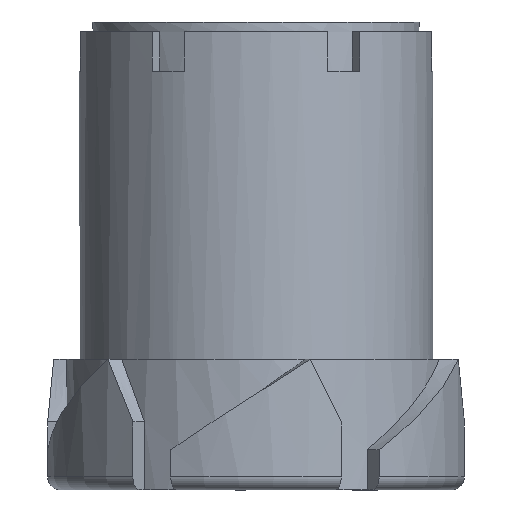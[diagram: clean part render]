
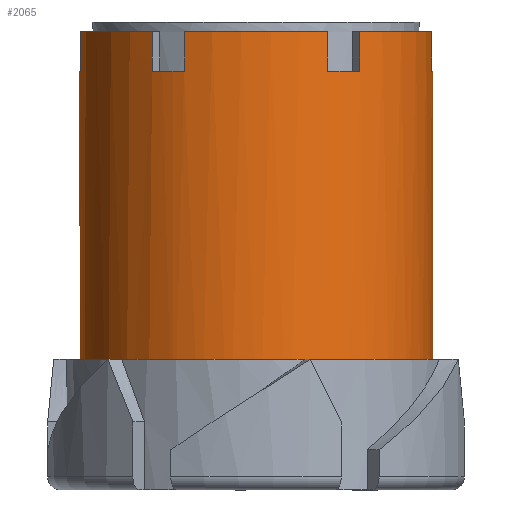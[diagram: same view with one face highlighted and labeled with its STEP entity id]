
A CAD part, left-side view. The second image highlights one B-rep face of the part: STEP entity #2065.
In plain terms, the highlighted cylindrical face has radius 27 mm (diameter 54 mm), a full revolution.
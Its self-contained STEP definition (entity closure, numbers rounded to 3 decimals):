
#1794=CARTESIAN_POINT('',(26.852,28.,-2.822));
#1795=VERTEX_POINT('',#1794);
#1802=CARTESIAN_POINT('',(26.852,34.0,-2.822));
#1803=VERTEX_POINT('',#1802);
#1804=CARTESIAN_POINT('',(26.852,34.0,-2.822));
#1805=DIRECTION('',(0.0,-1.0,0.0));
#1806=VECTOR('',#1805,6.);
#1807=LINE('',#1804,#1806);
#1808=EDGE_CURVE('',#1803,#1795,#1807,.T.);
#1833=CARTESIAN_POINT('',(15.87,34.0,-21.843));
#1834=VERTEX_POINT('',#1833);
#1835=CARTESIAN_POINT('',(0.0,34.0,0.0));
#1836=DIRECTION('',(0.0,-1.0,0.0));
#1837=DIRECTION('',(1.0,0.0,0.0));
#1838=AXIS2_PLACEMENT_3D('',#1835,#1836,#1837);
#1839=CIRCLE('',#1838,27.0);
#1840=EDGE_CURVE('',#1834,#1803,#1839,.T.);
#1860=CARTESIAN_POINT('',(0.0,0.0,0.0));
#1861=DIRECTION('',(0.0,1.0,0.0));
#1862=DIRECTION('',(1.0,0.0,0.0));
#1863=AXIS2_PLACEMENT_3D('',#1860,#1861,#1862);
#1864=CYLINDRICAL_SURFACE('',#1863,27.0);
#1865=CARTESIAN_POINT('',(-27.0,-36.0,0.));
#1866=VERTEX_POINT('',#1865);
#1867=CARTESIAN_POINT('',(0.0,-36.0,0.0));
#1868=DIRECTION('',(0.0,1.0,0.0));
#1869=DIRECTION('',(1.0,0.0,0.0));
#1870=AXIS2_PLACEMENT_3D('',#1867,#1868,#1869);
#1871=CIRCLE('',#1870,27.0);
#1872=EDGE_CURVE('',#1866,#1866,#1871,.T.);
#1873=ORIENTED_EDGE('',*,*,#1872,.T.);
#1874=EDGE_LOOP('',(#1873));
#1875=FACE_OUTER_BOUND('',#1874,.T.);
#1876=ORIENTED_EDGE('',*,*,#1808,.T.);
#1877=CARTESIAN_POINT('',(26.852,28.,2.822));
#1878=VERTEX_POINT('',#1877);
#1879=CARTESIAN_POINT('',(0.0,28.,0.0));
#1880=DIRECTION('',(0.0,-1.0,0.0));
#1881=DIRECTION('',(1.0,0.0,0.0));
#1882=AXIS2_PLACEMENT_3D('',#1879,#1880,#1881);
#1883=CIRCLE('',#1882,27.0);
#1884=EDGE_CURVE('',#1795,#1878,#1883,.T.);
#1885=ORIENTED_EDGE('',*,*,#1884,.T.);
#1886=CARTESIAN_POINT('',(26.852,34.0,2.822));
#1887=VERTEX_POINT('',#1886);
#1888=CARTESIAN_POINT('',(26.852,28.,2.822));
#1889=DIRECTION('',(0.0,1.0,0.0));
#1890=VECTOR('',#1889,6.);
#1891=LINE('',#1888,#1890);
#1892=EDGE_CURVE('',#1878,#1887,#1891,.T.);
#1893=ORIENTED_EDGE('',*,*,#1892,.T.);
#1894=CARTESIAN_POINT('',(15.87,34.0,21.843));
#1895=VERTEX_POINT('',#1894);
#1896=CARTESIAN_POINT('',(0.0,34.0,0.0));
#1897=DIRECTION('',(0.0,-1.0,0.0));
#1898=DIRECTION('',(1.0,0.0,0.0));
#1899=AXIS2_PLACEMENT_3D('',#1896,#1897,#1898);
#1900=CIRCLE('',#1899,27.0);
#1901=EDGE_CURVE('',#1887,#1895,#1900,.T.);
#1902=ORIENTED_EDGE('',*,*,#1901,.T.);
#1903=CARTESIAN_POINT('',(15.87,28.,21.843));
#1904=VERTEX_POINT('',#1903);
#1905=CARTESIAN_POINT('',(15.87,34.0,21.843));
#1906=DIRECTION('',(0.0,-1.0,0.0));
#1907=VECTOR('',#1906,6.);
#1908=LINE('',#1905,#1907);
#1909=EDGE_CURVE('',#1895,#1904,#1908,.T.);
#1910=ORIENTED_EDGE('',*,*,#1909,.T.);
#1911=CARTESIAN_POINT('',(10.982,28.,24.666));
#1912=VERTEX_POINT('',#1911);
#1913=CARTESIAN_POINT('',(0.0,28.,0.0));
#1914=DIRECTION('',(0.0,-1.0,0.0));
#1915=DIRECTION('',(1.0,0.0,0.0));
#1916=AXIS2_PLACEMENT_3D('',#1913,#1914,#1915);
#1917=CIRCLE('',#1916,27.0);
#1918=EDGE_CURVE('',#1904,#1912,#1917,.T.);
#1919=ORIENTED_EDGE('',*,*,#1918,.T.);
#1920=CARTESIAN_POINT('',(10.982,34.0,24.666));
#1921=VERTEX_POINT('',#1920);
#1922=CARTESIAN_POINT('',(10.982,28.,24.666));
#1923=DIRECTION('',(0.0,1.0,0.0));
#1924=VECTOR('',#1923,6.);
#1925=LINE('',#1922,#1924);
#1926=EDGE_CURVE('',#1912,#1921,#1925,.T.);
#1927=ORIENTED_EDGE('',*,*,#1926,.T.);
#1928=CARTESIAN_POINT('',(-10.982,34.0,24.666));
#1929=VERTEX_POINT('',#1928);
#1930=CARTESIAN_POINT('',(0.0,34.0,0.0));
#1931=DIRECTION('',(0.0,-1.0,0.0));
#1932=DIRECTION('',(1.0,0.0,0.0));
#1933=AXIS2_PLACEMENT_3D('',#1930,#1931,#1932);
#1934=CIRCLE('',#1933,27.0);
#1935=EDGE_CURVE('',#1921,#1929,#1934,.T.);
#1936=ORIENTED_EDGE('',*,*,#1935,.T.);
#1937=CARTESIAN_POINT('',(-10.982,28.,24.666));
#1938=VERTEX_POINT('',#1937);
#1939=CARTESIAN_POINT('',(-10.982,34.0,24.666));
#1940=DIRECTION('',(0.0,-1.0,0.0));
#1941=VECTOR('',#1940,6.);
#1942=LINE('',#1939,#1941);
#1943=EDGE_CURVE('',#1929,#1938,#1942,.T.);
#1944=ORIENTED_EDGE('',*,*,#1943,.T.);
#1945=CARTESIAN_POINT('',(-15.87,28.,21.843));
#1946=VERTEX_POINT('',#1945);
#1947=CARTESIAN_POINT('',(0.0,28.,0.0));
#1948=DIRECTION('',(0.0,-1.0,0.0));
#1949=DIRECTION('',(1.0,0.0,0.0));
#1950=AXIS2_PLACEMENT_3D('',#1947,#1948,#1949);
#1951=CIRCLE('',#1950,27.0);
#1952=EDGE_CURVE('',#1938,#1946,#1951,.T.);
#1953=ORIENTED_EDGE('',*,*,#1952,.T.);
#1954=CARTESIAN_POINT('',(-15.87,34.0,21.843));
#1955=VERTEX_POINT('',#1954);
#1956=CARTESIAN_POINT('',(-15.87,28.,21.843));
#1957=DIRECTION('',(0.0,1.0,0.0));
#1958=VECTOR('',#1957,6.);
#1959=LINE('',#1956,#1958);
#1960=EDGE_CURVE('',#1946,#1955,#1959,.T.);
#1961=ORIENTED_EDGE('',*,*,#1960,.T.);
#1962=CARTESIAN_POINT('',(-26.852,34.0,2.822));
#1963=VERTEX_POINT('',#1962);
#1964=CARTESIAN_POINT('',(0.0,34.0,0.0));
#1965=DIRECTION('',(0.0,-1.0,0.0));
#1966=DIRECTION('',(1.0,0.0,0.0));
#1967=AXIS2_PLACEMENT_3D('',#1964,#1965,#1966);
#1968=CIRCLE('',#1967,27.0);
#1969=EDGE_CURVE('',#1955,#1963,#1968,.T.);
#1970=ORIENTED_EDGE('',*,*,#1969,.T.);
#1971=CARTESIAN_POINT('',(-26.852,28.,2.822));
#1972=VERTEX_POINT('',#1971);
#1973=CARTESIAN_POINT('',(-26.852,34.0,2.822));
#1974=DIRECTION('',(0.0,-1.0,0.0));
#1975=VECTOR('',#1974,6.);
#1976=LINE('',#1973,#1975);
#1977=EDGE_CURVE('',#1963,#1972,#1976,.T.);
#1978=ORIENTED_EDGE('',*,*,#1977,.T.);
#1979=CARTESIAN_POINT('',(-26.852,28.,-2.822));
#1980=VERTEX_POINT('',#1979);
#1981=CARTESIAN_POINT('',(0.0,28.,0.0));
#1982=DIRECTION('',(0.0,-1.0,0.0));
#1983=DIRECTION('',(1.0,0.0,0.0));
#1984=AXIS2_PLACEMENT_3D('',#1981,#1982,#1983);
#1985=CIRCLE('',#1984,27.0);
#1986=EDGE_CURVE('',#1972,#1980,#1985,.T.);
#1987=ORIENTED_EDGE('',*,*,#1986,.T.);
#1988=CARTESIAN_POINT('',(-26.852,34.0,-2.822));
#1989=VERTEX_POINT('',#1988);
#1990=CARTESIAN_POINT('',(-26.852,28.,-2.822));
#1991=DIRECTION('',(0.0,1.0,0.0));
#1992=VECTOR('',#1991,6.);
#1993=LINE('',#1990,#1992);
#1994=EDGE_CURVE('',#1980,#1989,#1993,.T.);
#1995=ORIENTED_EDGE('',*,*,#1994,.T.);
#1996=CARTESIAN_POINT('',(-15.87,34.0,-21.843));
#1997=VERTEX_POINT('',#1996);
#1998=CARTESIAN_POINT('',(0.0,34.0,0.0));
#1999=DIRECTION('',(0.0,-1.0,0.0));
#2000=DIRECTION('',(1.0,0.0,0.0));
#2001=AXIS2_PLACEMENT_3D('',#1998,#1999,#2000);
#2002=CIRCLE('',#2001,27.0);
#2003=EDGE_CURVE('',#1989,#1997,#2002,.T.);
#2004=ORIENTED_EDGE('',*,*,#2003,.T.);
#2005=CARTESIAN_POINT('',(-15.87,28.,-21.843));
#2006=VERTEX_POINT('',#2005);
#2007=CARTESIAN_POINT('',(-15.87,34.0,-21.843));
#2008=DIRECTION('',(0.0,-1.0,0.0));
#2009=VECTOR('',#2008,6.);
#2010=LINE('',#2007,#2009);
#2011=EDGE_CURVE('',#1997,#2006,#2010,.T.);
#2012=ORIENTED_EDGE('',*,*,#2011,.T.);
#2013=CARTESIAN_POINT('',(-10.982,28.,-24.666));
#2014=VERTEX_POINT('',#2013);
#2015=CARTESIAN_POINT('',(0.0,28.,0.0));
#2016=DIRECTION('',(0.0,-1.0,0.0));
#2017=DIRECTION('',(1.0,0.0,0.0));
#2018=AXIS2_PLACEMENT_3D('',#2015,#2016,#2017);
#2019=CIRCLE('',#2018,27.0);
#2020=EDGE_CURVE('',#2006,#2014,#2019,.T.);
#2021=ORIENTED_EDGE('',*,*,#2020,.T.);
#2022=CARTESIAN_POINT('',(-10.982,34.0,-24.666));
#2023=VERTEX_POINT('',#2022);
#2024=CARTESIAN_POINT('',(-10.982,28.,-24.666));
#2025=DIRECTION('',(0.0,1.0,0.0));
#2026=VECTOR('',#2025,6.);
#2027=LINE('',#2024,#2026);
#2028=EDGE_CURVE('',#2014,#2023,#2027,.T.);
#2029=ORIENTED_EDGE('',*,*,#2028,.T.);
#2030=CARTESIAN_POINT('',(10.982,34.0,-24.666));
#2031=VERTEX_POINT('',#2030);
#2032=CARTESIAN_POINT('',(0.0,34.0,0.0));
#2033=DIRECTION('',(0.0,-1.0,0.0));
#2034=DIRECTION('',(1.0,0.0,0.0));
#2035=AXIS2_PLACEMENT_3D('',#2032,#2033,#2034);
#2036=CIRCLE('',#2035,27.0);
#2037=EDGE_CURVE('',#2023,#2031,#2036,.T.);
#2038=ORIENTED_EDGE('',*,*,#2037,.T.);
#2039=CARTESIAN_POINT('',(10.982,28.,-24.666));
#2040=VERTEX_POINT('',#2039);
#2041=CARTESIAN_POINT('',(10.982,34.0,-24.666));
#2042=DIRECTION('',(0.0,-1.0,0.0));
#2043=VECTOR('',#2042,6.);
#2044=LINE('',#2041,#2043);
#2045=EDGE_CURVE('',#2031,#2040,#2044,.T.);
#2046=ORIENTED_EDGE('',*,*,#2045,.T.);
#2047=CARTESIAN_POINT('',(15.87,28.,-21.843));
#2048=VERTEX_POINT('',#2047);
#2049=CARTESIAN_POINT('',(0.0,28.,0.0));
#2050=DIRECTION('',(0.0,-1.0,0.0));
#2051=DIRECTION('',(1.0,0.0,0.0));
#2052=AXIS2_PLACEMENT_3D('',#2049,#2050,#2051);
#2053=CIRCLE('',#2052,27.0);
#2054=EDGE_CURVE('',#2040,#2048,#2053,.T.);
#2055=ORIENTED_EDGE('',*,*,#2054,.T.);
#2056=CARTESIAN_POINT('',(15.87,28.,-21.843));
#2057=DIRECTION('',(0.0,1.0,0.0));
#2058=VECTOR('',#2057,6.);
#2059=LINE('',#2056,#2058);
#2060=EDGE_CURVE('',#2048,#1834,#2059,.T.);
#2061=ORIENTED_EDGE('',*,*,#2060,.T.);
#2062=ORIENTED_EDGE('',*,*,#1840,.T.);
#2063=EDGE_LOOP('',(#1876,#1885,#1893,#1902,#1910,#1919,#1927,#1936,#1944,#1953,#1961,#1970,#1978,#1987,#1995,#2004,#2012,#2021,#2029,#2038,#2046,#2055,#2061,#2062));
#2064=FACE_BOUND('',#2063,.T.);
#2065=ADVANCED_FACE('',(#1875,#2064),#1864,.T.);
